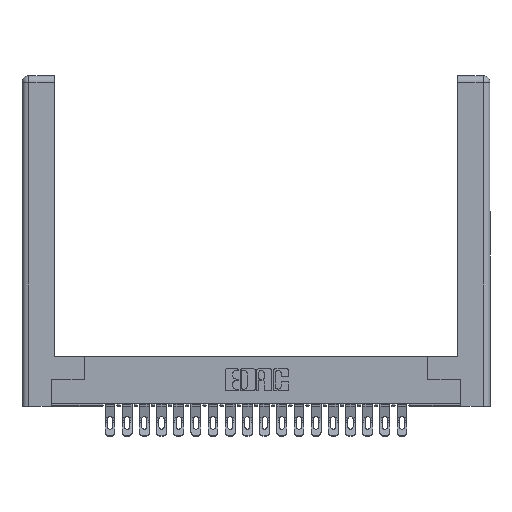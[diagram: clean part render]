
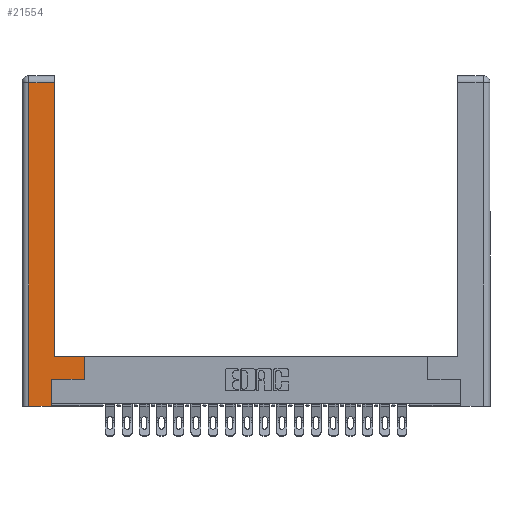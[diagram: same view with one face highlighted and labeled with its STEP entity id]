
A CAD part, top view. The second image highlights one B-rep face of the part: STEP entity #21554.
In plain terms, the highlighted planar face has unit normal (0, 0, 1).
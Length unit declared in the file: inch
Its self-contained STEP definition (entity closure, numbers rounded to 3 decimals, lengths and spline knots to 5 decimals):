
#556 = ORIENTED_EDGE ( 'NONE', *, *, #17349, .T. ) ;
#1087 = CARTESIAN_POINT ( 'NONE',  ( 0.565, 0.45, 0. ) ) ;
#1167 = EDGE_CURVE ( 'NONE', #9124, #14363, #2811, .T. ) ;
#1518 = VECTOR ( 'NONE', #6921, 39.37008 ) ;
#1885 = FACE_OUTER_BOUND ( 'NONE', #17036, .T. ) ;
#2129 = DIRECTION ( 'NONE',  ( -1., 0., 0. ) ) ;
#2177 = VERTEX_POINT ( 'NONE', #13458 ) ;
#2317 = DIRECTION ( 'NONE',  ( -1., 0., 0. ) ) ;
#2681 = LINE ( 'NONE', #17125, #11319 ) ;
#2811 = LINE ( 'NONE', #9415, #25406 ) ;
#3021 = VERTEX_POINT ( 'NONE', #1087 ) ;
#3302 = VERTEX_POINT ( 'NONE', #24247 ) ;
#4164 = DIRECTION ( 'NONE',  ( 0., 1., 0. ) ) ;
#4308 = AXIS2_PLACEMENT_3D ( 'NONE', #19916, #14165, #2317 ) ;
#4577 = CARTESIAN_POINT ( 'NONE',  ( 0.295, 2.94, 0. ) ) ;
#5086 = LINE ( 'NONE', #6238, #16495 ) ;
#5467 = EDGE_CURVE ( 'NONE', #2177, #11918, #18822, .T. ) ;
#6238 = CARTESIAN_POINT ( 'NONE',  ( 0.295, 3., 0. ) ) ;
#6921 = DIRECTION ( 'NONE',  ( 0., -1., 0. ) ) ;
#7462 = ORIENTED_EDGE ( 'NONE', *, *, #11049, .T. ) ;
#9124 = VERTEX_POINT ( 'NONE', #4577 ) ;
#9411 = EDGE_CURVE ( 'NONE', #3302, #3021, #23735, .T. ) ;
#9415 = CARTESIAN_POINT ( 'NONE',  ( 0.0615, 2.94, 0. ) ) ;
#9958 = EDGE_CURVE ( 'NONE', #18996, #2177, #2681, .T. ) ;
#11049 = EDGE_CURVE ( 'NONE', #3021, #18195, #21494, .T. ) ;
#11319 = VECTOR ( 'NONE', #14950, 39.37008 ) ;
#11788 = DIRECTION ( 'NONE',  ( -1., 0., 0. ) ) ;
#11918 = VERTEX_POINT ( 'NONE', #21361 ) ;
#12264 = CARTESIAN_POINT ( 'NONE',  ( 0.565, 0.245, 0. ) ) ;
#12333 = CARTESIAN_POINT ( 'NONE',  ( 0.295, 0.45, 0. ) ) ;
#12342 = CARTESIAN_POINT ( 'NONE',  ( 0.265, 0.245, 0. ) ) ;
#13458 = CARTESIAN_POINT ( 'NONE',  ( 0.265, 0., 0. ) ) ;
#14047 = DIRECTION ( 'NONE',  ( 0., 1., 0. ) ) ;
#14134 = EDGE_CURVE ( 'NONE', #14363, #18996, #22570, .T. ) ;
#14165 = DIRECTION ( 'NONE',  ( 0., 0., -1. ) ) ;
#14363 = VERTEX_POINT ( 'NONE', #25512 ) ;
#14416 = DIRECTION ( 'NONE',  ( 0., 1., 0. ) ) ;
#14489 = ORIENTED_EDGE ( 'NONE', *, *, #19935, .T. ) ;
#14950 = DIRECTION ( 'NONE',  ( 1., 0., 0. ) ) ;
#15667 = LINE ( 'NONE', #12264, #25604 ) ;
#16152 = PLANE ( 'NONE',  #4308 ) ;
#16495 = VECTOR ( 'NONE', #4164, 39.37008 ) ;
#17036 = EDGE_LOOP ( 'NONE', ( #14489, #24723, #18354, #19948, #20791, #556, #20460, #7462 ) ) ;
#17125 = CARTESIAN_POINT ( 'NONE',  ( 0.265, 0., 0. ) ) ;
#17349 = EDGE_CURVE ( 'NONE', #11918, #3302, #15667, .T. ) ;
#17900 = DIRECTION ( 'NONE',  ( 1., 0., 0. ) ) ;
#18195 = VERTEX_POINT ( 'NONE', #19091 ) ;
#18354 = ORIENTED_EDGE ( 'NONE', *, *, #14134, .T. ) ;
#18822 = LINE ( 'NONE', #12342, #19453 ) ;
#18996 = VERTEX_POINT ( 'NONE', #22636 ) ;
#19091 = CARTESIAN_POINT ( 'NONE',  ( 0.295, 0.45, 0. ) ) ;
#19453 = VECTOR ( 'NONE', #14416, 39.37008 ) ;
#19748 = VECTOR ( 'NONE', #14047, 39.37008 ) ;
#19916 = CARTESIAN_POINT ( 'NONE',  ( 0., 0., 0. ) ) ;
#19935 = EDGE_CURVE ( 'NONE', #18195, #9124, #5086, .T. ) ;
#19948 = ORIENTED_EDGE ( 'NONE', *, *, #9958, .T. ) ;
#20043 = CARTESIAN_POINT ( 'NONE',  ( 0.565, 0.45, 0. ) ) ;
#20460 = ORIENTED_EDGE ( 'NONE', *, *, #9411, .T. ) ;
#20791 = ORIENTED_EDGE ( 'NONE', *, *, #5467, .T. ) ;
#21361 = CARTESIAN_POINT ( 'NONE',  ( 0.265, 0.245, 0. ) ) ;
#21494 = LINE ( 'NONE', #12333, #22714 ) ;
#21554 = ADVANCED_FACE ( 'NONE', ( #1885 ), #16152, .F. ) ;
#22570 = LINE ( 'NONE', #24547, #1518 ) ;
#22636 = CARTESIAN_POINT ( 'NONE',  ( 0.0615, 0., 0. ) ) ;
#22714 = VECTOR ( 'NONE', #2129, 39.37008 ) ;
#23735 = LINE ( 'NONE', #20043, #19748 ) ;
#24247 = CARTESIAN_POINT ( 'NONE',  ( 0.565, 0.245, 0. ) ) ;
#24547 = CARTESIAN_POINT ( 'NONE',  ( 0.0615, 0., 0. ) ) ;
#24723 = ORIENTED_EDGE ( 'NONE', *, *, #1167, .T. ) ;
#25406 = VECTOR ( 'NONE', #11788, 39.37008 ) ;
#25512 = CARTESIAN_POINT ( 'NONE',  ( 0.0615, 2.94, 0. ) ) ;
#25604 = VECTOR ( 'NONE', #17900, 39.37008 ) ;
